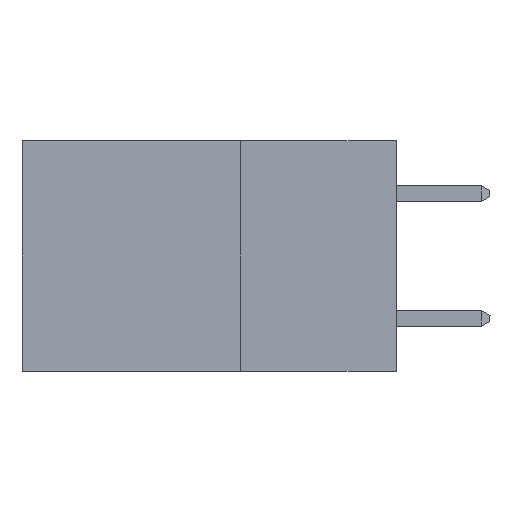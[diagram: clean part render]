
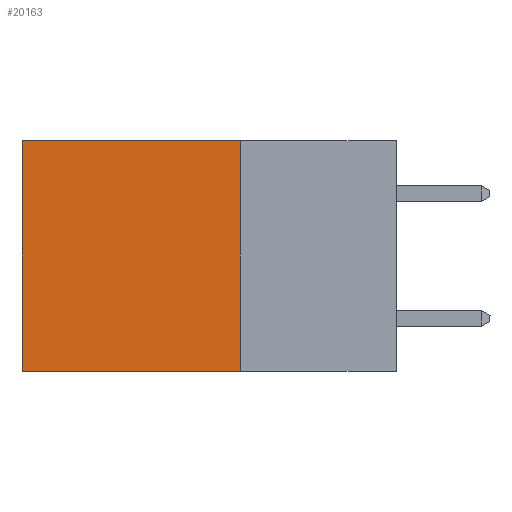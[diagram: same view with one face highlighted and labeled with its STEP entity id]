
A CAD part, left-side view. The second image highlights one B-rep face of the part: STEP entity #20163.
In plain terms, the highlighted planar face has unit normal (-1, 0, 0).
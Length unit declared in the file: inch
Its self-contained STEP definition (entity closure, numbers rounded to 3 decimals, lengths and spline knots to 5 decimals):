
#190 = VERTEX_POINT ( 'NONE', #7974 ) ;
#240 = VECTOR ( 'NONE', #10884, 39.37008 ) ;
#2784 = CARTESIAN_POINT ( 'NONE',  ( 0.298, 0.6, -0.37 ) ) ;
#3434 = FACE_OUTER_BOUND ( 'NONE', #9135, .T. ) ;
#4516 = DIRECTION ( 'NONE',  ( 0., 1., 0. ) ) ;
#5309 = EDGE_CURVE ( 'NONE', #14280, #6078, #7643, .T. ) ;
#5704 = VECTOR ( 'NONE', #7200, 39.37008 ) ;
#5878 = DIRECTION ( 'NONE',  ( 0., 0., -1. ) ) ;
#6078 = VERTEX_POINT ( 'NONE', #2784 ) ;
#6435 = LINE ( 'NONE', #16259, #5704 ) ;
#6844 = ORIENTED_EDGE ( 'NONE', *, *, #5309, .F. ) ;
#6949 = PLANE ( 'NONE',  #16716 ) ;
#7200 = DIRECTION ( 'NONE',  ( 0., 0., -1. ) ) ;
#7332 = LINE ( 'NONE', #19883, #16586 ) ;
#7526 = EDGE_CURVE ( 'NONE', #17066, #14280, #7332, .T. ) ;
#7643 = LINE ( 'NONE', #13822, #11814 ) ;
#7776 = EDGE_CURVE ( 'NONE', #17066, #190, #13701, .T. ) ;
#7974 = CARTESIAN_POINT ( 'NONE',  ( 0.298, 0.6, 0. ) ) ;
#9014 = CARTESIAN_POINT ( 'NONE',  ( 0.298, 0.25, 0. ) ) ;
#9135 = EDGE_LOOP ( 'NONE', ( #20182, #6844, #14823, #10585 ) ) ;
#10406 = EDGE_CURVE ( 'NONE', #190, #6078, #6435, .T. ) ;
#10585 = ORIENTED_EDGE ( 'NONE', *, *, #7776, .T. ) ;
#10884 = DIRECTION ( 'NONE',  ( 0., 1., 0. ) ) ;
#11814 = VECTOR ( 'NONE', #4516, 39.37008 ) ;
#12072 = CARTESIAN_POINT ( 'NONE',  ( 0.298, 0.25, -0.37 ) ) ;
#12959 = DIRECTION ( 'NONE',  ( 1., 0., 0. ) ) ;
#13701 = LINE ( 'NONE', #18720, #240 ) ;
#13822 = CARTESIAN_POINT ( 'NONE',  ( 0.298, 0.25, -0.37 ) ) ;
#14280 = VERTEX_POINT ( 'NONE', #12072 ) ;
#14823 = ORIENTED_EDGE ( 'NONE', *, *, #7526, .F. ) ;
#16207 = CARTESIAN_POINT ( 'NONE',  ( 0.298, 0.25, 0. ) ) ;
#16259 = CARTESIAN_POINT ( 'NONE',  ( 0.298, 0.6, 0. ) ) ;
#16586 = VECTOR ( 'NONE', #5878, 39.37008 ) ;
#16716 = AXIS2_PLACEMENT_3D ( 'NONE', #16207, #12959, #19351 ) ;
#17066 = VERTEX_POINT ( 'NONE', #9014 ) ;
#18720 = CARTESIAN_POINT ( 'NONE',  ( 0.298, 0.25, 0. ) ) ;
#19351 = DIRECTION ( 'NONE',  ( 0., 0., -1. ) ) ;
#19883 = CARTESIAN_POINT ( 'NONE',  ( 0.298, 0.25, 0. ) ) ;
#20163 = ADVANCED_FACE ( 'NONE', ( #3434 ), #6949, .F. ) ;
#20182 = ORIENTED_EDGE ( 'NONE', *, *, #10406, .T. ) ;
